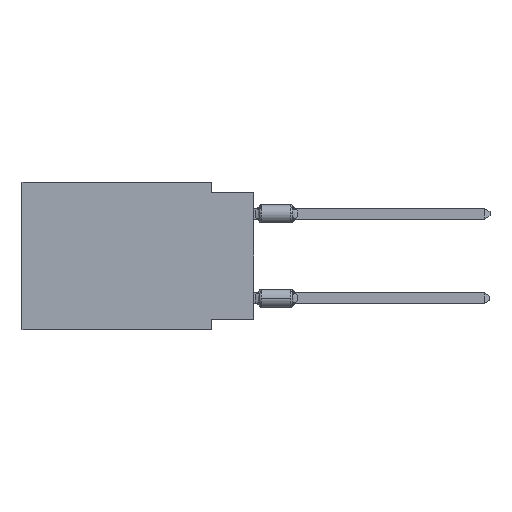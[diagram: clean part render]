
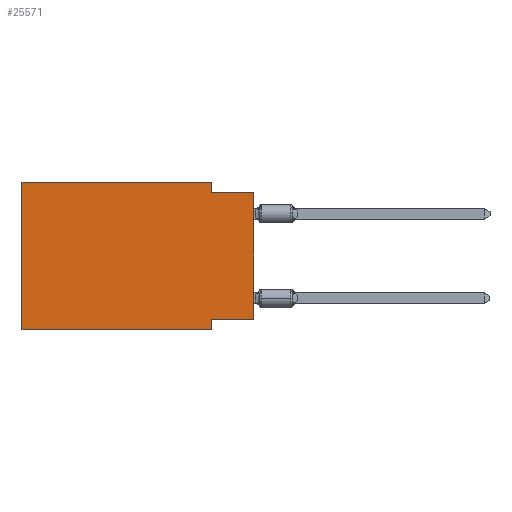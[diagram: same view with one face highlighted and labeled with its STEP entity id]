
A CAD part, left-side view. The second image highlights one B-rep face of the part: STEP entity #25571.
In plain terms, the highlighted planar face has unit normal (-1, 0, 0).
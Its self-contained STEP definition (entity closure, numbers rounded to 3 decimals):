
#152 = VECTOR ( 'NONE', #18231, 1000. ) ;
#358 = CARTESIAN_POINT ( 'NONE',  ( 0., 2.54, -8.89 ) ) ;
#1458 = VECTOR ( 'NONE', #3367, 1000. ) ;
#3367 = DIRECTION ( 'NONE',  ( 0., -1., 0. ) ) ;
#3688 = CARTESIAN_POINT ( 'NONE',  ( 0., 2.54, -8.89 ) ) ;
#4249 = LINE ( 'NONE', #35946, #31901 ) ;
#4285 = EDGE_CURVE ( 'NONE', #17833, #22743, #38454, .T. ) ;
#5765 = LINE ( 'NONE', #3688, #22659 ) ;
#5787 = DIRECTION ( 'NONE',  ( 0., 0., -1. ) ) ;
#6804 = EDGE_CURVE ( 'NONE', #24393, #25180, #4249, .T. ) ;
#7853 = CARTESIAN_POINT ( 'NONE',  ( 0., 13.97, 0. ) ) ;
#10217 = LINE ( 'NONE', #16055, #1458 ) ;
#10250 = CARTESIAN_POINT ( 'NONE',  ( 0., 0., -8.255 ) ) ;
#10834 = LINE ( 'NONE', #10250, #11537 ) ;
#11537 = VECTOR ( 'NONE', #35147, 1000. ) ;
#11988 = LINE ( 'NONE', #24283, #152 ) ;
#12257 = EDGE_CURVE ( 'NONE', #39171, #32081, #5765, .T. ) ;
#12306 = EDGE_CURVE ( 'NONE', #35142, #25180, #11988, .T. ) ;
#13203 = CARTESIAN_POINT ( 'NONE',  ( 0., 2.54, -8.255 ) ) ;
#14699 = ORIENTED_EDGE ( 'NONE', *, *, #6804, .T. ) ;
#15961 = DIRECTION ( 'NONE',  ( 0., 0., -1. ) ) ;
#16055 = CARTESIAN_POINT ( 'NONE',  ( 0., 13.97, 0. ) ) ;
#16469 = VECTOR ( 'NONE', #16948, 1000. ) ;
#16948 = DIRECTION ( 'NONE',  ( 0., 0., 1. ) ) ;
#17472 = CARTESIAN_POINT ( 'NONE',  ( 0., 13.97, -8.89 ) ) ;
#17814 = ORIENTED_EDGE ( 'NONE', *, *, #26040, .F. ) ;
#17833 = VERTEX_POINT ( 'NONE', #17472 ) ;
#18231 = DIRECTION ( 'NONE',  ( 0., -1., 0. ) ) ;
#18607 = ORIENTED_EDGE ( 'NONE', *, *, #24597, .F. ) ;
#19316 = CARTESIAN_POINT ( 'NONE',  ( 0., 0., -8.255 ) ) ;
#19551 = DIRECTION ( 'NONE',  ( 0., 0., -1. ) ) ;
#20277 = EDGE_LOOP ( 'NONE', ( #14699, #25599, #18607, #31124, #39407, #39084, #28351, #17814 ) ) ;
#22296 = CARTESIAN_POINT ( 'NONE',  ( 0., 13.97, -8.89 ) ) ;
#22659 = VECTOR ( 'NONE', #15961, 1000. ) ;
#22743 = VERTEX_POINT ( 'NONE', #38195 ) ;
#23169 = FACE_OUTER_BOUND ( 'NONE', #20277, .T. ) ;
#24283 = CARTESIAN_POINT ( 'NONE',  ( 0., 0., -0.635 ) ) ;
#24363 = AXIS2_PLACEMENT_3D ( 'NONE', #7853, #35587, #19551 ) ;
#24393 = VERTEX_POINT ( 'NONE', #19316 ) ;
#24506 = LINE ( 'NONE', #24699, #36050 ) ;
#24597 = EDGE_CURVE ( 'NONE', #24826, #35142, #24506, .T. ) ;
#24699 = CARTESIAN_POINT ( 'NONE',  ( 0., 2.54, 0. ) ) ;
#24826 = VERTEX_POINT ( 'NONE', #28317 ) ;
#24925 = LINE ( 'NONE', #22296, #25247 ) ;
#25180 = VERTEX_POINT ( 'NONE', #35046 ) ;
#25247 = VECTOR ( 'NONE', #31133, 1000. ) ;
#25571 = ADVANCED_FACE ( 'NONE', ( #23169 ), #32001, .F. ) ;
#25599 = ORIENTED_EDGE ( 'NONE', *, *, #12306, .F. ) ;
#25651 = CARTESIAN_POINT ( 'NONE',  ( 0., 2.54, -0.635 ) ) ;
#26040 = EDGE_CURVE ( 'NONE', #24393, #39171, #10834, .T. ) ;
#28317 = CARTESIAN_POINT ( 'NONE',  ( 0., 2.54, 0. ) ) ;
#28351 = ORIENTED_EDGE ( 'NONE', *, *, #12257, .F. ) ;
#31124 = ORIENTED_EDGE ( 'NONE', *, *, #32073, .F. ) ;
#31133 = DIRECTION ( 'NONE',  ( 0., -1., 0. ) ) ;
#31901 = VECTOR ( 'NONE', #34805, 1000. ) ;
#32001 = PLANE ( 'NONE',  #24363 ) ;
#32073 = EDGE_CURVE ( 'NONE', #22743, #24826, #10217, .T. ) ;
#32081 = VERTEX_POINT ( 'NONE', #358 ) ;
#32109 = EDGE_CURVE ( 'NONE', #17833, #32081, #24925, .T. ) ;
#34805 = DIRECTION ( 'NONE',  ( 0., 0., 1. ) ) ;
#35046 = CARTESIAN_POINT ( 'NONE',  ( 0., 0., -0.635 ) ) ;
#35142 = VERTEX_POINT ( 'NONE', #25651 ) ;
#35147 = DIRECTION ( 'NONE',  ( 0., 1., 0. ) ) ;
#35587 = DIRECTION ( 'NONE',  ( 1., 0., 0. ) ) ;
#35946 = CARTESIAN_POINT ( 'NONE',  ( 0., 0., 0. ) ) ;
#36050 = VECTOR ( 'NONE', #5787, 1000. ) ;
#38195 = CARTESIAN_POINT ( 'NONE',  ( 0., 13.97, 0. ) ) ;
#38252 = CARTESIAN_POINT ( 'NONE',  ( 0., 13.97, 0. ) ) ;
#38454 = LINE ( 'NONE', #38252, #16469 ) ;
#39084 = ORIENTED_EDGE ( 'NONE', *, *, #32109, .T. ) ;
#39171 = VERTEX_POINT ( 'NONE', #13203 ) ;
#39407 = ORIENTED_EDGE ( 'NONE', *, *, #4285, .F. ) ;
